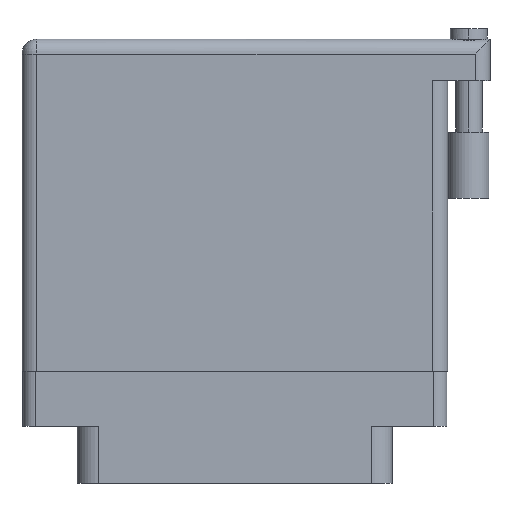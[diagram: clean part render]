
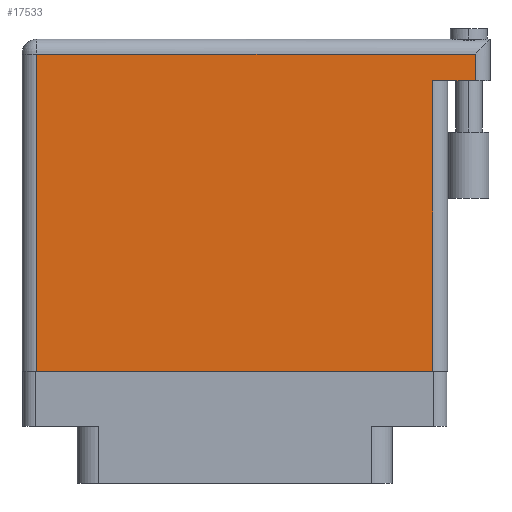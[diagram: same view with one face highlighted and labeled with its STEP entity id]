
A CAD part, front view. The second image highlights one B-rep face of the part: STEP entity #17533.
In plain terms, the highlighted face is planar.
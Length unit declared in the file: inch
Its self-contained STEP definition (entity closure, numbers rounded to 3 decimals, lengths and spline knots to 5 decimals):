
#60 = VECTOR ( 'NONE', #22879, 39.37008 ) ;
#912 = VERTEX_POINT ( 'NONE', #22910 ) ;
#1238 = EDGE_CURVE ( 'NONE', #27492, #912, #32358, .T. ) ;
#1392 = DIRECTION ( 'NONE',  ( 0., -1., 0. ) ) ;
#1638 = VERTEX_POINT ( 'NONE', #33411 ) ;
#1781 = VECTOR ( 'NONE', #33882, 39.37008 ) ;
#1856 = ORIENTED_EDGE ( 'NONE', *, *, #13705, .T. ) ;
#2179 = EDGE_LOOP ( 'NONE', ( #1856, #8797, #27315, #22112, #6100, #15676 ) ) ;
#2430 = CARTESIAN_POINT ( 'NONE',  ( 1.938, 0., 0. ) ) ;
#2484 = EDGE_CURVE ( 'NONE', #27492, #19864, #7158, .T. ) ;
#2800 = EDGE_CURVE ( 'NONE', #9291, #912, #7983, .T. ) ;
#4563 = FACE_OUTER_BOUND ( 'NONE', #2179, .T. ) ;
#4734 = CARTESIAN_POINT ( 'NONE',  ( 0., 0., 0. ) ) ;
#6100 = ORIENTED_EDGE ( 'NONE', *, *, #9894, .T. ) ;
#7158 = LINE ( 'NONE', #19766, #1781 ) ;
#7272 = PLANE ( 'NONE',  #20810 ) ;
#7983 = LINE ( 'NONE', #8241, #23508 ) ;
#8241 = CARTESIAN_POINT ( 'NONE',  ( 1.938, 1.369, 0. ) ) ;
#8797 = ORIENTED_EDGE ( 'NONE', *, *, #2800, .T. ) ;
#9291 = VERTEX_POINT ( 'NONE', #2430 ) ;
#9894 = EDGE_CURVE ( 'NONE', #19864, #32953, #28124, .T. ) ;
#13705 = EDGE_CURVE ( 'NONE', #1638, #9291, #20904, .T. ) ;
#13786 = VECTOR ( 'NONE', #23464, 39.37008 ) ;
#15676 = ORIENTED_EDGE ( 'NONE', *, *, #17469, .T. ) ;
#15994 = CARTESIAN_POINT ( 'NONE',  ( 2.208, 1.369, 0. ) ) ;
#17469 = EDGE_CURVE ( 'NONE', #32953, #1638, #28843, .T. ) ;
#17533 = ADVANCED_FACE ( 'NONE', ( #4563 ), #7272, .F. ) ;
#19766 = CARTESIAN_POINT ( 'NONE',  ( 2.138, 1.566, 0. ) ) ;
#19864 = VERTEX_POINT ( 'NONE', #23509 ) ;
#20810 = AXIS2_PLACEMENT_3D ( 'NONE', #23240, #34194, #33851 ) ;
#20904 = LINE ( 'NONE', #4734, #13786 ) ;
#21494 = DIRECTION ( 'NONE',  ( 0., 1., 0. ) ) ;
#22112 = ORIENTED_EDGE ( 'NONE', *, *, #2484, .T. ) ;
#22653 = CARTESIAN_POINT ( 'NONE',  ( 0.07, 0., 0. ) ) ;
#22879 = DIRECTION ( 'NONE',  ( -1., 0., 0. ) ) ;
#22910 = CARTESIAN_POINT ( 'NONE',  ( 1.938, 1.369, 0. ) ) ;
#23240 = CARTESIAN_POINT ( 'NONE',  ( 0., 1.566, 0. ) ) ;
#23464 = DIRECTION ( 'NONE',  ( 1., 0., 0. ) ) ;
#23508 = VECTOR ( 'NONE', #21494, 39.37008 ) ;
#23509 = CARTESIAN_POINT ( 'NONE',  ( 2.138, 1.496, 0. ) ) ;
#24919 = CARTESIAN_POINT ( 'NONE',  ( 2.138, 1.369, 0. ) ) ;
#25568 = CARTESIAN_POINT ( 'NONE',  ( 0., 1.496, 0. ) ) ;
#25930 = VECTOR ( 'NONE', #1392, 39.37008 ) ;
#26521 = DIRECTION ( 'NONE',  ( -1., 0., 0. ) ) ;
#27226 = CARTESIAN_POINT ( 'NONE',  ( 0.07, 1.496, 0. ) ) ;
#27315 = ORIENTED_EDGE ( 'NONE', *, *, #1238, .F. ) ;
#27492 = VERTEX_POINT ( 'NONE', #24919 ) ;
#28124 = LINE ( 'NONE', #25568, #60 ) ;
#28843 = LINE ( 'NONE', #22653, #25930 ) ;
#32358 = LINE ( 'NONE', #15994, #33601 ) ;
#32953 = VERTEX_POINT ( 'NONE', #27226 ) ;
#33411 = CARTESIAN_POINT ( 'NONE',  ( 0.07, 0., 0. ) ) ;
#33601 = VECTOR ( 'NONE', #26521, 39.37008 ) ;
#33851 = DIRECTION ( 'NONE',  ( -1., 0., 0. ) ) ;
#33882 = DIRECTION ( 'NONE',  ( 0., 1., 0. ) ) ;
#34194 = DIRECTION ( 'NONE',  ( 0., 0., -1. ) ) ;
